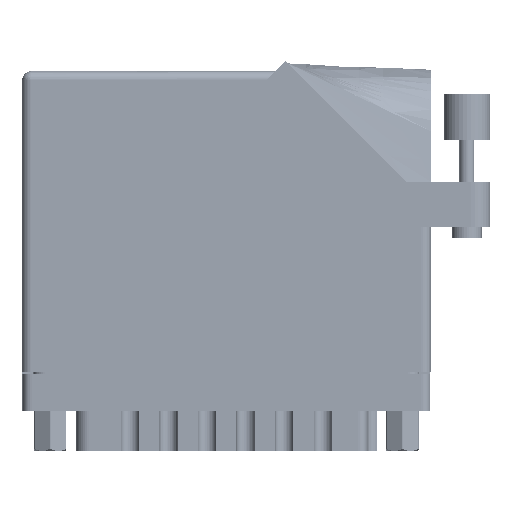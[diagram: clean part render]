
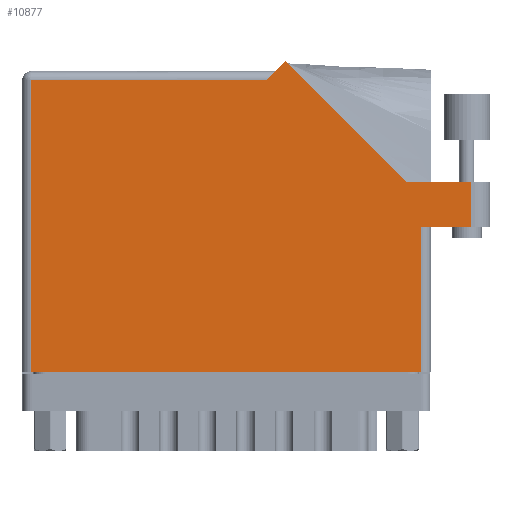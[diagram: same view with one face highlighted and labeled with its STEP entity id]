
A CAD part, front view. The second image highlights one B-rep face of the part: STEP entity #10877.
In plain terms, the highlighted face is planar.
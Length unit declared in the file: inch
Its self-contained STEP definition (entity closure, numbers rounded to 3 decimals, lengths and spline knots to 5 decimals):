
#243 = ORIENTED_EDGE ( 'NONE', *, *, #49645, .T. ) ;
#622 = EDGE_CURVE ( 'NONE', #78944, #39662, #74087, .T. ) ;
#1518 = EDGE_CURVE ( 'NONE', #74935, #33645, #70046, .T. ) ;
#1669 = CARTESIAN_POINT ( 'NONE',  ( 0.062, 0., 0. ) ) ;
#2531 = ORIENTED_EDGE ( 'NONE', *, *, #89871, .T. ) ;
#8419 = LINE ( 'NONE', #68742, #67413 ) ;
#8727 = DIRECTION ( 'NONE',  ( 0., 1., 0. ) ) ;
#9504 = CARTESIAN_POINT ( 'NONE',  ( 0., 0., 0. ) ) ;
#9908 = VECTOR ( 'NONE', #88194, 39.37008 ) ;
#10877 = ADVANCED_FACE ( 'NONE', ( #45894 ), #53577, .F. ) ;
#16158 = DIRECTION ( 'NONE',  ( 0., 1., 0. ) ) ;
#16215 = LINE ( 'NONE', #9504, #76512 ) ;
#17384 = CARTESIAN_POINT ( 'NONE',  ( 0.062, 0., 0. ) ) ;
#19087 = CARTESIAN_POINT ( 'NONE',  ( 2.755, 0.98, 0. ) ) ;
#19998 = CARTESIAN_POINT ( 'NONE',  ( 1.77571, 2.10071, 0. ) ) ;
#23807 = DIRECTION ( 'NONE',  ( 0., 0., -1. ) ) ;
#30878 = CARTESIAN_POINT ( 'NONE',  ( 2.58942, 1.287, 0. ) ) ;
#31915 = EDGE_CURVE ( 'NONE', #37122, #78944, #37424, .T. ) ;
#33645 = VERTEX_POINT ( 'NONE', #17384 ) ;
#36637 = CARTESIAN_POINT ( 'NONE',  ( 2.693, 0.98, 0. ) ) ;
#37122 = VERTEX_POINT ( 'NONE', #96825 ) ;
#37424 = LINE ( 'NONE', #80716, #86184 ) ;
#38416 = CARTESIAN_POINT ( 'NONE',  ( 2.693, 0., 0. ) ) ;
#39662 = VERTEX_POINT ( 'NONE', #104424 ) ;
#40275 = CARTESIAN_POINT ( 'NONE',  ( 2.693, 0.98, 0. ) ) ;
#40306 = CARTESIAN_POINT ( 'NONE',  ( 0., 2.03, 0. ) ) ;
#40592 = AXIS2_PLACEMENT_3D ( 'NONE', #40306, #23807, #63597 ) ;
#45894 = FACE_OUTER_BOUND ( 'NONE', #56382, .T. ) ;
#46422 = VECTOR ( 'NONE', #55949, 39.37008 ) ;
#46977 = ORIENTED_EDGE ( 'NONE', *, *, #1518, .T. ) ;
#49219 = DIRECTION ( 'NONE',  ( 0., -1., 0. ) ) ;
#49645 = EDGE_CURVE ( 'NONE', #94029, #99923, #87491, .T. ) ;
#50709 = ORIENTED_EDGE ( 'NONE', *, *, #88554, .T. ) ;
#53577 = PLANE ( 'NONE',  #40592 ) ;
#55949 = DIRECTION ( 'NONE',  ( -1., 0., 0. ) ) ;
#56382 = EDGE_LOOP ( 'NONE', ( #2531, #69418, #72579, #50709, #63022, #99285, #46977, #65517, #243 ) ) ;
#63022 = ORIENTED_EDGE ( 'NONE', *, *, #74470, .T. ) ;
#63597 = DIRECTION ( 'NONE',  ( -1., 0., 0. ) ) ;
#65517 = ORIENTED_EDGE ( 'NONE', *, *, #81098, .T. ) ;
#67413 = VECTOR ( 'NONE', #101908, 39.37008 ) ;
#67421 = VECTOR ( 'NONE', #84349, 39.37008 ) ;
#68742 = CARTESIAN_POINT ( 'NONE',  ( 1.705, 2.03, 0. ) ) ;
#69418 = ORIENTED_EDGE ( 'NONE', *, *, #31915, .T. ) ;
#70046 = LINE ( 'NONE', #1669, #71296 ) ;
#70790 = VECTOR ( 'NONE', #8727, 39.37008 ) ;
#71296 = VECTOR ( 'NONE', #49219, 39.37008 ) ;
#72579 = ORIENTED_EDGE ( 'NONE', *, *, #622, .T. ) ;
#73346 = CARTESIAN_POINT ( 'NONE',  ( 3.03, 1.287, 0. ) ) ;
#73422 = LINE ( 'NONE', #87196, #46422 ) ;
#74087 = LINE ( 'NONE', #88466, #90751 ) ;
#74470 = EDGE_CURVE ( 'NONE', #103201, #104769, #8419, .T. ) ;
#74935 = VERTEX_POINT ( 'NONE', #87831 ) ;
#76512 = VECTOR ( 'NONE', #82270, 39.37008 ) ;
#77704 = LINE ( 'NONE', #19087, #67421 ) ;
#78944 = VERTEX_POINT ( 'NONE', #73346 ) ;
#80664 = CARTESIAN_POINT ( 'NONE',  ( 1.643, 1.968, 0. ) ) ;
#80716 = CARTESIAN_POINT ( 'NONE',  ( 3.03, 1.287, 0. ) ) ;
#81098 = EDGE_CURVE ( 'NONE', #33645, #94029, #16215, .T. ) ;
#82270 = DIRECTION ( 'NONE',  ( 1., 0., 0. ) ) ;
#84349 = DIRECTION ( 'NONE',  ( 1., 0., 0. ) ) ;
#86184 = VECTOR ( 'NONE', #16158, 39.37008 ) ;
#87196 = CARTESIAN_POINT ( 'NONE',  ( 0., 1.968, 0. ) ) ;
#87491 = LINE ( 'NONE', #40275, #70790 ) ;
#87831 = CARTESIAN_POINT ( 'NONE',  ( 0.062, 1.968, 0. ) ) ;
#88194 = DIRECTION ( 'NONE',  ( -0.707, 0.707, 0. ) ) ;
#88466 = CARTESIAN_POINT ( 'NONE',  ( 3.155, 1.287, 0. ) ) ;
#88554 = EDGE_CURVE ( 'NONE', #39662, #103201, #90739, .T. ) ;
#89871 = EDGE_CURVE ( 'NONE', #99923, #37122, #77704, .T. ) ;
#90739 = LINE ( 'NONE', #30878, #9908 ) ;
#90751 = VECTOR ( 'NONE', #97106, 39.37008 ) ;
#92888 = EDGE_CURVE ( 'NONE', #104769, #74935, #73422, .T. ) ;
#94029 = VERTEX_POINT ( 'NONE', #38416 ) ;
#96825 = CARTESIAN_POINT ( 'NONE',  ( 3.03, 0.98, 0. ) ) ;
#97106 = DIRECTION ( 'NONE',  ( -1., 0., 0. ) ) ;
#99285 = ORIENTED_EDGE ( 'NONE', *, *, #92888, .T. ) ;
#99923 = VERTEX_POINT ( 'NONE', #36637 ) ;
#101908 = DIRECTION ( 'NONE',  ( -0.707, -0.707, 0. ) ) ;
#103201 = VERTEX_POINT ( 'NONE', #19998 ) ;
#104424 = CARTESIAN_POINT ( 'NONE',  ( 2.58942, 1.287, 0. ) ) ;
#104769 = VERTEX_POINT ( 'NONE', #80664 ) ;
